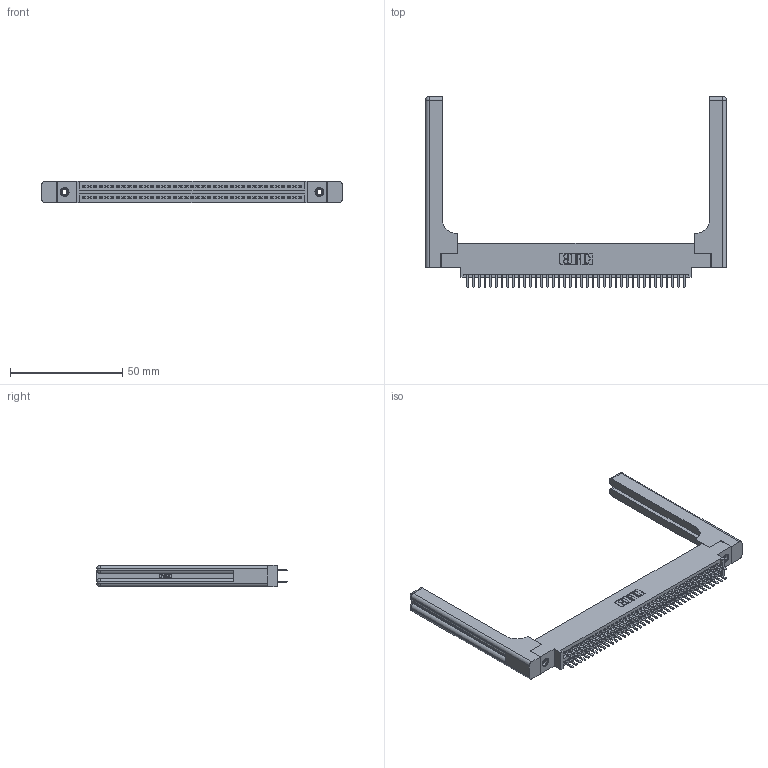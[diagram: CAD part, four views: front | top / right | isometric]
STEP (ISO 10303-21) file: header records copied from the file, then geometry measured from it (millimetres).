
FILE_DESCRIPTION (( 'STEP AP203' ), '1' );
FILE_NAME ('395-078-520-858.STEP', '2019-10-24T18:16:30', ( '' ), ( '' ), 'SwSTEP 2.0', 'SolidWorks 2016', '' );
FILE_SCHEMA (( 'CONFIG_CONTROL_DESIGN' ));
Length unit declared in the file: inch
Products named in the file (5): 395-078-520-858; 345 Part_0.170 Offset - 0.156 Dia-TH; 345-292-001_345-293-120; 345-250-001_345-250-001-102; 345-220-058_345-220-058
Assembly tree (83 placements, depth 2):
  395-078-520-858
    345 Part_0.170 Offset - 0.156 Dia-TH
    345-292-001_345-293-120  x78
    345-250-001_345-250-001-102  x2
    345-220-058_345-220-058  x2
Bounding box: 134.09 x 84.96 x 9.4 mm (x, y, z)
Volume: 21324.9 mm3; surface area: 24065.4 mm2
Topology: 83 solids, 83 shells, 4598 faces, 13265 edges, 8614 vertices
Faces by surface type: plane 2962, cylinder 1576, bspline 36, cone 12, sphere 8, torus 4
Entity records: 36432 total; most frequent: CARTESIAN_POINT 7117, ORIENTED_EDGE 5836, DIRECTION 5198, EDGE_CURVE 2918, VECTOR 2534, LINE 2534, VERTEX_POINT 1934, AXIS2_PLACEMENT_3D 1332
